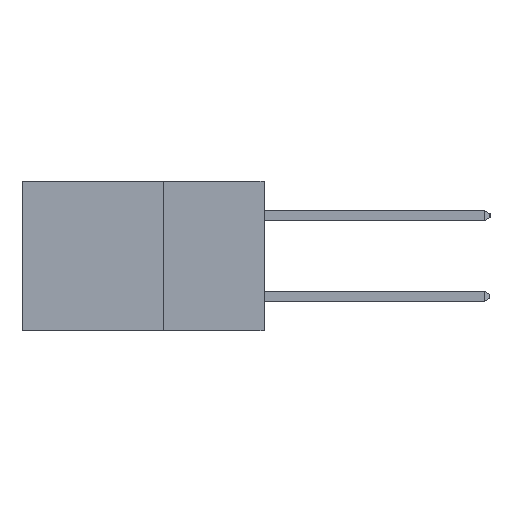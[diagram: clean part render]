
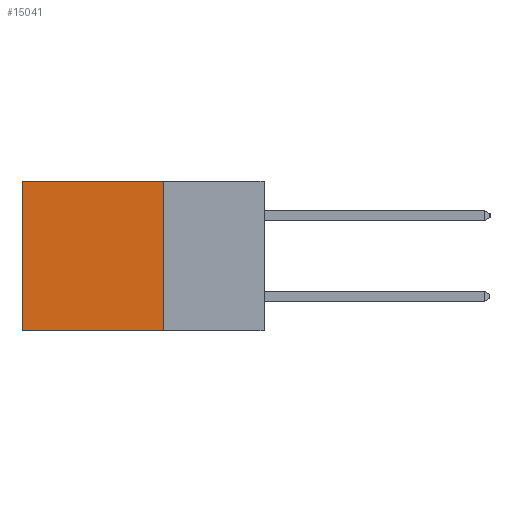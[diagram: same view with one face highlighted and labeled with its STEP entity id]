
A CAD part, left-side view. The second image highlights one B-rep face of the part: STEP entity #15041.
In plain terms, the highlighted planar face has unit normal (-1, 0, 0).
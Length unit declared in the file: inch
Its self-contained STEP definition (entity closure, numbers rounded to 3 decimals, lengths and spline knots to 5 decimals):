
#291 = VECTOR ( 'NONE', #13531, 39.37008 ) ;
#594 = VERTEX_POINT ( 'NONE', #15356 ) ;
#2411 = VERTEX_POINT ( 'NONE', #6577 ) ;
#2549 = FACE_OUTER_BOUND ( 'NONE', #3200, .T. ) ;
#2992 = LINE ( 'NONE', #10340, #11473 ) ;
#3200 = EDGE_LOOP ( 'NONE', ( #7983, #11980, #15069, #9008 ) ) ;
#3416 = VERTEX_POINT ( 'NONE', #5802 ) ;
#3825 = CARTESIAN_POINT ( 'NONE',  ( 0.2615, 0.25, -0.37 ) ) ;
#4055 = VECTOR ( 'NONE', #9733, 39.37008 ) ;
#4558 = LINE ( 'NONE', #9431, #4055 ) ;
#4848 = EDGE_CURVE ( 'NONE', #13660, #594, #11143, .T. ) ;
#5215 = LINE ( 'NONE', #10087, #13487 ) ;
#5802 = CARTESIAN_POINT ( 'NONE',  ( 0.2615, 0.6, -0.37 ) ) ;
#6102 = EDGE_CURVE ( 'NONE', #13660, #2411, #4558, .T. ) ;
#6577 = CARTESIAN_POINT ( 'NONE',  ( 0.2615, 0.6, 0. ) ) ;
#7405 = PLANE ( 'NONE',  #11096 ) ;
#7912 = EDGE_CURVE ( 'NONE', #594, #3416, #5215, .T. ) ;
#7983 = ORIENTED_EDGE ( 'NONE', *, *, #8813, .T. ) ;
#8699 = DIRECTION ( 'NONE',  ( 0., 0., -1. ) ) ;
#8813 = EDGE_CURVE ( 'NONE', #2411, #3416, #2992, .T. ) ;
#9008 = ORIENTED_EDGE ( 'NONE', *, *, #6102, .T. ) ;
#9259 = CARTESIAN_POINT ( 'NONE',  ( 0.2615, 0.25, 0. ) ) ;
#9431 = CARTESIAN_POINT ( 'NONE',  ( 0.2615, 0.25, 0. ) ) ;
#9733 = DIRECTION ( 'NONE',  ( 0., 1., 0. ) ) ;
#10087 = CARTESIAN_POINT ( 'NONE',  ( 0.2615, 0.25, -0.37 ) ) ;
#10340 = CARTESIAN_POINT ( 'NONE',  ( 0.2615, 0.6, -0.37 ) ) ;
#11096 = AXIS2_PLACEMENT_3D ( 'NONE', #3825, #11168, #8699 ) ;
#11143 = LINE ( 'NONE', #12335, #291 ) ;
#11168 = DIRECTION ( 'NONE',  ( 1., 0., 0. ) ) ;
#11210 = DIRECTION ( 'NONE',  ( 0., 1., 0. ) ) ;
#11473 = VECTOR ( 'NONE', #12731, 39.37008 ) ;
#11980 = ORIENTED_EDGE ( 'NONE', *, *, #7912, .F. ) ;
#12335 = CARTESIAN_POINT ( 'NONE',  ( 0.2615, 0.25, -0.37 ) ) ;
#12731 = DIRECTION ( 'NONE',  ( 0., 0., -1. ) ) ;
#13487 = VECTOR ( 'NONE', #11210, 39.37008 ) ;
#13531 = DIRECTION ( 'NONE',  ( 0., 0., -1. ) ) ;
#13660 = VERTEX_POINT ( 'NONE', #9259 ) ;
#15041 = ADVANCED_FACE ( 'NONE', ( #2549 ), #7405, .F. ) ;
#15069 = ORIENTED_EDGE ( 'NONE', *, *, #4848, .F. ) ;
#15356 = CARTESIAN_POINT ( 'NONE',  ( 0.2615, 0.25, -0.37 ) ) ;
